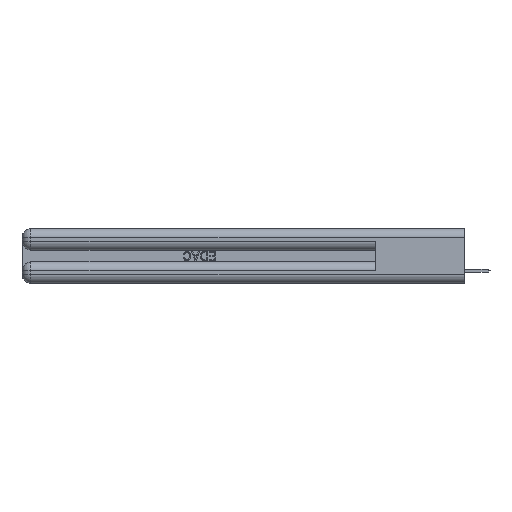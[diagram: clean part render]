
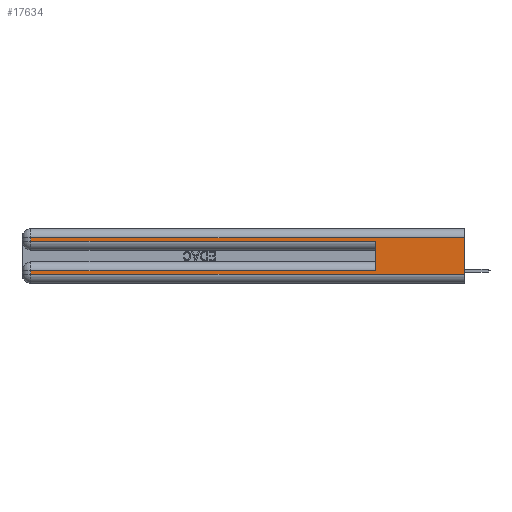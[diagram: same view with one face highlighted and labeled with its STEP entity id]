
A CAD part, left-side view. The second image highlights one B-rep face of the part: STEP entity #17634.
In plain terms, the highlighted planar face has unit normal (-1, 0, 0).
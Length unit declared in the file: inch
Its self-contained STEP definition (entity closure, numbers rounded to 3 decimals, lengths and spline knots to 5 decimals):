
#3453 = VERTEX_POINT ( 'NONE', #15803 ) ;
#5909 = VERTEX_POINT ( 'NONE', #8827 ) ;
#6505 = LINE ( 'NONE', #26649, #7004 ) ;
#7004 = VECTOR ( 'NONE', #26049, 39.37008 ) ;
#7187 = LINE ( 'NONE', #27465, #24027 ) ;
#8360 = DIRECTION ( 'NONE',  ( 0., 1., 0. ) ) ;
#8692 = EDGE_CURVE ( 'NONE', #3453, #27397, #12631, .T. ) ;
#8773 = CARTESIAN_POINT ( 'NONE',  ( 0., 0., 0.31 ) ) ;
#8827 = CARTESIAN_POINT ( 'NONE',  ( 0., 0., 0.31 ) ) ;
#9349 = VERTEX_POINT ( 'NONE', #22346 ) ;
#9469 = EDGE_LOOP ( 'NONE', ( #22006, #22290, #38629, #23270, #21360, #33690, #29068, #39556 ) ) ;
#9782 = DIRECTION ( 'NONE',  ( 0., 0., -1. ) ) ;
#11135 = EDGE_CURVE ( 'NONE', #20068, #31700, #31004, .T. ) ;
#11344 = CARTESIAN_POINT ( 'NONE',  ( 0., 0.6, 0.285 ) ) ;
#12631 = LINE ( 'NONE', #29594, #15798 ) ;
#12714 = PLANE ( 'NONE',  #42034 ) ;
#12912 = CARTESIAN_POINT ( 'NONE',  ( 0., 0.6, 0.145 ) ) ;
#14843 = CARTESIAN_POINT ( 'NONE',  ( 0., 0.6, 0.085 ) ) ;
#15798 = VECTOR ( 'NONE', #35683, 39.37008 ) ;
#15803 = CARTESIAN_POINT ( 'NONE',  ( 0., 2.94, 0.06 ) ) ;
#16000 = VECTOR ( 'NONE', #19678, 39.37008 ) ;
#16114 = CARTESIAN_POINT ( 'NONE',  ( 0., 0., 0.37 ) ) ;
#16197 = VECTOR ( 'NONE', #29212, 39.37008 ) ;
#17634 = ADVANCED_FACE ( 'NONE', ( #29367 ), #12714, .F. ) ;
#18345 = EDGE_CURVE ( 'NONE', #22955, #9349, #42483, .T. ) ;
#18735 = EDGE_CURVE ( 'NONE', #5909, #27397, #7187, .T. ) ;
#19291 = VECTOR ( 'NONE', #8360, 39.37008 ) ;
#19564 = VERTEX_POINT ( 'NONE', #11344 ) ;
#19678 = DIRECTION ( 'NONE',  ( 0., 0., 1. ) ) ;
#20068 = VERTEX_POINT ( 'NONE', #24429 ) ;
#21360 = ORIENTED_EDGE ( 'NONE', *, *, #28524, .F. ) ;
#21809 = CARTESIAN_POINT ( 'NONE',  ( 0., 2.94, 0.37 ) ) ;
#22006 = ORIENTED_EDGE ( 'NONE', *, *, #18735, .F. ) ;
#22290 = ORIENTED_EDGE ( 'NONE', *, *, #41757, .T. ) ;
#22346 = CARTESIAN_POINT ( 'NONE',  ( 0., 2.94, 0.085 ) ) ;
#22955 = VERTEX_POINT ( 'NONE', #14843 ) ;
#23270 = ORIENTED_EDGE ( 'NONE', *, *, #25994, .T. ) ;
#23536 = DIRECTION ( 'NONE',  ( 0., 0., -1. ) ) ;
#24027 = VECTOR ( 'NONE', #23536, 39.37008 ) ;
#24429 = CARTESIAN_POINT ( 'NONE',  ( 0., 2.94, 0.31 ) ) ;
#25131 = VECTOR ( 'NONE', #25208, 39.37008 ) ;
#25208 = DIRECTION ( 'NONE',  ( 0., 0., -1. ) ) ;
#25994 = EDGE_CURVE ( 'NONE', #31700, #19564, #6505, .T. ) ;
#26049 = DIRECTION ( 'NONE',  ( 0., -1., 0. ) ) ;
#26649 = CARTESIAN_POINT ( 'NONE',  ( 0., 0., 0.285 ) ) ;
#27397 = VERTEX_POINT ( 'NONE', #30767 ) ;
#27465 = CARTESIAN_POINT ( 'NONE',  ( 0., 0., 0.37 ) ) ;
#27740 = LINE ( 'NONE', #8773, #16197 ) ;
#28514 = CARTESIAN_POINT ( 'NONE',  ( 0., 0., 0.085 ) ) ;
#28524 = EDGE_CURVE ( 'NONE', #22955, #19564, #33602, .T. ) ;
#28660 = DIRECTION ( 'NONE',  ( 0., 0., -1. ) ) ;
#29068 = ORIENTED_EDGE ( 'NONE', *, *, #41689, .T. ) ;
#29212 = DIRECTION ( 'NONE',  ( 0., 1., 0. ) ) ;
#29367 = FACE_OUTER_BOUND ( 'NONE', #9469, .T. ) ;
#29594 = CARTESIAN_POINT ( 'NONE',  ( 0., 0., 0.06 ) ) ;
#29912 = DIRECTION ( 'NONE',  ( 1., 0., 0. ) ) ;
#30767 = CARTESIAN_POINT ( 'NONE',  ( 0., 0., 0.06 ) ) ;
#31004 = LINE ( 'NONE', #35411, #41074 ) ;
#31700 = VERTEX_POINT ( 'NONE', #42399 ) ;
#33602 = LINE ( 'NONE', #12912, #16000 ) ;
#33690 = ORIENTED_EDGE ( 'NONE', *, *, #18345, .T. ) ;
#35411 = CARTESIAN_POINT ( 'NONE',  ( 0., 2.94, 0.37 ) ) ;
#35683 = DIRECTION ( 'NONE',  ( 0., -1., 0. ) ) ;
#36676 = LINE ( 'NONE', #21809, #25131 ) ;
#38629 = ORIENTED_EDGE ( 'NONE', *, *, #11135, .T. ) ;
#39556 = ORIENTED_EDGE ( 'NONE', *, *, #8692, .T. ) ;
#41074 = VECTOR ( 'NONE', #28660, 39.37008 ) ;
#41689 = EDGE_CURVE ( 'NONE', #9349, #3453, #36676, .T. ) ;
#41757 = EDGE_CURVE ( 'NONE', #5909, #20068, #27740, .T. ) ;
#42034 = AXIS2_PLACEMENT_3D ( 'NONE', #16114, #29912, #9782 ) ;
#42399 = CARTESIAN_POINT ( 'NONE',  ( 0., 2.94, 0.285 ) ) ;
#42483 = LINE ( 'NONE', #28514, #19291 ) ;
